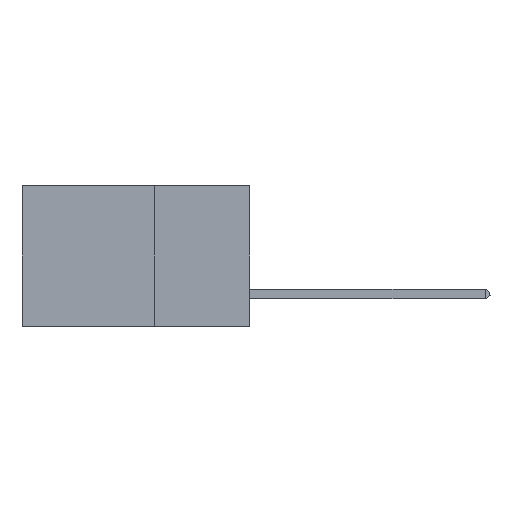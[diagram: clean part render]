
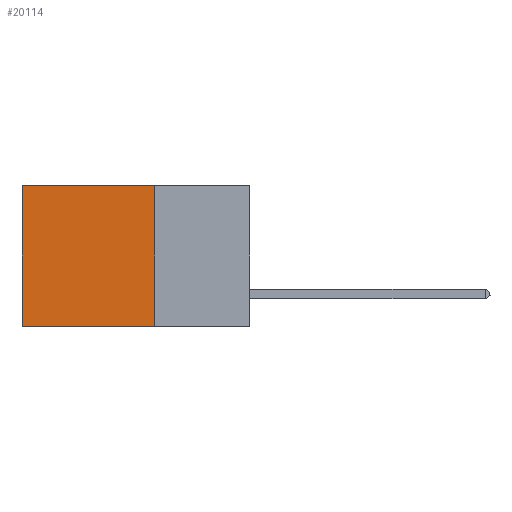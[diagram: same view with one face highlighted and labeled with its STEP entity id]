
A CAD part, left-side view. The second image highlights one B-rep face of the part: STEP entity #20114.
In plain terms, the highlighted planar face has unit normal (-1, 0, 0).
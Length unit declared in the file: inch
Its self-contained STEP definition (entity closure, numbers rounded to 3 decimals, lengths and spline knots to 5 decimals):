
#305 = ORIENTED_EDGE ( 'NONE', *, *, #7463, .F. ) ;
#326 = VERTEX_POINT ( 'NONE', #7604 ) ;
#1970 = DIRECTION ( 'NONE',  ( 0., 0., -1. ) ) ;
#2620 = VERTEX_POINT ( 'NONE', #10846 ) ;
#2739 = LINE ( 'NONE', #26640, #16572 ) ;
#3452 = CARTESIAN_POINT ( 'NONE',  ( 0.2875, 0.25, 0. ) ) ;
#3724 = CARTESIAN_POINT ( 'NONE',  ( 0.2875, 0.25, -0.37 ) ) ;
#4299 = CARTESIAN_POINT ( 'NONE',  ( 0.2875, 0.25, 0. ) ) ;
#5803 = DIRECTION ( 'NONE',  ( 0., 1., 0. ) ) ;
#7329 = VECTOR ( 'NONE', #5803, 39.37008 ) ;
#7463 = EDGE_CURVE ( 'NONE', #16562, #326, #23449, .T. ) ;
#7604 = CARTESIAN_POINT ( 'NONE',  ( 0.2875, 0.6, -0.37 ) ) ;
#8095 = CARTESIAN_POINT ( 'NONE',  ( 0.2875, 0.6, 0. ) ) ;
#8797 = DIRECTION ( 'NONE',  ( 0., 1., 0. ) ) ;
#8815 = ORIENTED_EDGE ( 'NONE', *, *, #9073, .T. ) ;
#8924 = LINE ( 'NONE', #8095, #11533 ) ;
#9073 = EDGE_CURVE ( 'NONE', #2620, #326, #8924, .T. ) ;
#9158 = VECTOR ( 'NONE', #8797, 39.37008 ) ;
#9951 = DIRECTION ( 'NONE',  ( 0., 0., -1. ) ) ;
#10846 = CARTESIAN_POINT ( 'NONE',  ( 0.2875, 0.6, 0. ) ) ;
#11533 = VECTOR ( 'NONE', #9951, 39.37008 ) ;
#11765 = AXIS2_PLACEMENT_3D ( 'NONE', #25280, #19178, #1970 ) ;
#13131 = EDGE_CURVE ( 'NONE', #16465, #16562, #2739, .T. ) ;
#14784 = LINE ( 'NONE', #4299, #9158 ) ;
#16465 = VERTEX_POINT ( 'NONE', #3452 ) ;
#16562 = VERTEX_POINT ( 'NONE', #3724 ) ;
#16572 = VECTOR ( 'NONE', #26354, 39.37008 ) ;
#17781 = FACE_OUTER_BOUND ( 'NONE', #21779, .T. ) ;
#18796 = EDGE_CURVE ( 'NONE', #16465, #2620, #14784, .T. ) ;
#19129 = ORIENTED_EDGE ( 'NONE', *, *, #13131, .F. ) ;
#19178 = DIRECTION ( 'NONE',  ( 1., 0., 0. ) ) ;
#20114 = ADVANCED_FACE ( 'NONE', ( #17781 ), #23064, .F. ) ;
#21779 = EDGE_LOOP ( 'NONE', ( #8815, #305, #19129, #27132 ) ) ;
#23064 = PLANE ( 'NONE',  #11765 ) ;
#23449 = LINE ( 'NONE', #26917, #7329 ) ;
#25280 = CARTESIAN_POINT ( 'NONE',  ( 0.2875, 0.25, 0. ) ) ;
#26354 = DIRECTION ( 'NONE',  ( 0., 0., -1. ) ) ;
#26640 = CARTESIAN_POINT ( 'NONE',  ( 0.2875, 0.25, 0. ) ) ;
#26917 = CARTESIAN_POINT ( 'NONE',  ( 0.2875, 0.25, -0.37 ) ) ;
#27132 = ORIENTED_EDGE ( 'NONE', *, *, #18796, .T. ) ;
